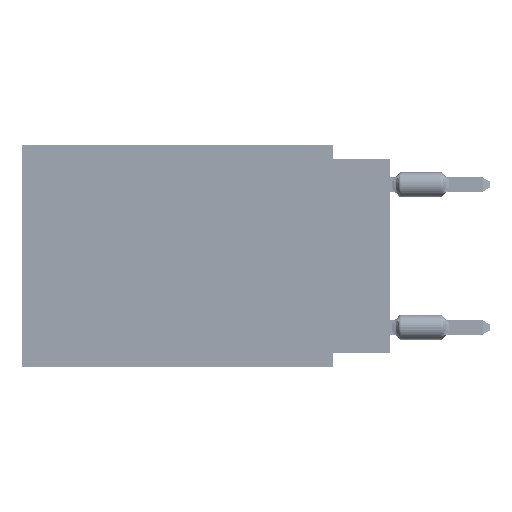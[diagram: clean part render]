
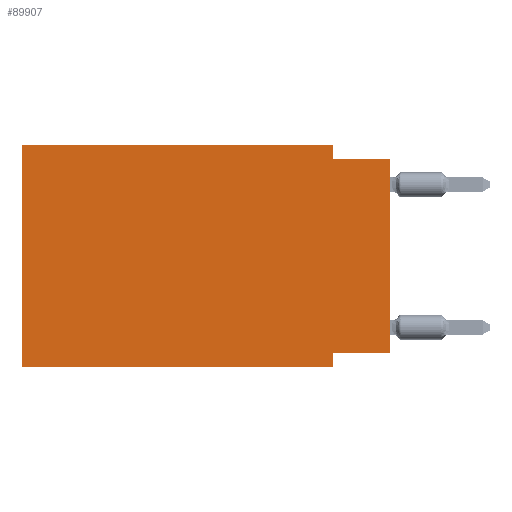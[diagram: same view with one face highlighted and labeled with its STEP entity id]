
A CAD part, left-side view. The second image highlights one B-rep face of the part: STEP entity #89907.
In plain terms, the highlighted planar face has unit normal (-1, 0, 0).
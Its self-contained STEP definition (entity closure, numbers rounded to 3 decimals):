
#1405 = LINE ( 'NONE', #71544, #45225 ) ;
#1411 = CARTESIAN_POINT ( 'NONE',  ( 0., 2.54, -9.906 ) ) ;
#1851 = AXIS2_PLACEMENT_3D ( 'NONE', #86816, #78167, #9817 ) ;
#9817 = DIRECTION ( 'NONE',  ( 0., 0., -1. ) ) ;
#9855 = ORIENTED_EDGE ( 'NONE', *, *, #84044, .T. ) ;
#11608 = ORIENTED_EDGE ( 'NONE', *, *, #20546, .T. ) ;
#14075 = VERTEX_POINT ( 'NONE', #1411 ) ;
#14467 = DIRECTION ( 'NONE',  ( 0., 0., 1. ) ) ;
#15139 = VECTOR ( 'NONE', #46938, 1000. ) ;
#15737 = VERTEX_POINT ( 'NONE', #35145 ) ;
#16542 = ORIENTED_EDGE ( 'NONE', *, *, #52613, .F. ) ;
#17741 = LINE ( 'NONE', #72874, #49326 ) ;
#18715 = LINE ( 'NONE', #19161, #15139 ) ;
#19161 = CARTESIAN_POINT ( 'NONE',  ( 0., 2.54, 0. ) ) ;
#20546 = EDGE_CURVE ( 'NONE', #51513, #14075, #88664, .T. ) ;
#20823 = VERTEX_POINT ( 'NONE', #58097 ) ;
#21518 = DIRECTION ( 'NONE',  ( 0., 0., -1. ) ) ;
#21965 = LINE ( 'NONE', #42917, #78584 ) ;
#22818 = EDGE_CURVE ( 'NONE', #60749, #85610, #1405, .T. ) ;
#23262 = DIRECTION ( 'NONE',  ( 0., -1., 0. ) ) ;
#26639 = VERTEX_POINT ( 'NONE', #79595 ) ;
#27002 = CARTESIAN_POINT ( 'NONE',  ( 0., 16.383, 0. ) ) ;
#28291 = ORIENTED_EDGE ( 'NONE', *, *, #59258, .F. ) ;
#28511 = CARTESIAN_POINT ( 'NONE',  ( 0., 2.54, -0.635 ) ) ;
#30251 = EDGE_LOOP ( 'NONE', ( #9855, #84826, #80996, #77245, #28291, #11608, #16542, #58809 ) ) ;
#33290 = VECTOR ( 'NONE', #14467, 1000. ) ;
#33835 = LINE ( 'NONE', #27002, #82146 ) ;
#35109 = CARTESIAN_POINT ( 'NONE',  ( 0., 16.383, 0. ) ) ;
#35145 = CARTESIAN_POINT ( 'NONE',  ( 0., 0., -9.271 ) ) ;
#42917 = CARTESIAN_POINT ( 'NONE',  ( 0., 2.54, -9.906 ) ) ;
#45225 = VECTOR ( 'NONE', #23262, 1000. ) ;
#46938 = DIRECTION ( 'NONE',  ( 0., 0., -1. ) ) ;
#49326 = VECTOR ( 'NONE', #59668, 1000. ) ;
#50366 = FACE_OUTER_BOUND ( 'NONE', #30251, .T. ) ;
#50719 = DIRECTION ( 'NONE',  ( 0., -1., 0. ) ) ;
#51172 = CARTESIAN_POINT ( 'NONE',  ( 0., 16.383, 0. ) ) ;
#51513 = VERTEX_POINT ( 'NONE', #52484 ) ;
#51613 = LINE ( 'NONE', #51172, #52098 ) ;
#52098 = VECTOR ( 'NONE', #50719, 1000. ) ;
#52484 = CARTESIAN_POINT ( 'NONE',  ( 0., 16.383, -9.906 ) ) ;
#52613 = EDGE_CURVE ( 'NONE', #26639, #14075, #21965, .T. ) ;
#54063 = CARTESIAN_POINT ( 'NONE',  ( 0., 0., -0.635 ) ) ;
#54790 = DIRECTION ( 'NONE',  ( 0., 0., 1. ) ) ;
#57299 = LINE ( 'NONE', #63220, #33290 ) ;
#58097 = CARTESIAN_POINT ( 'NONE',  ( 0., 2.54, 0. ) ) ;
#58809 = ORIENTED_EDGE ( 'NONE', *, *, #66293, .F. ) ;
#59258 = EDGE_CURVE ( 'NONE', #51513, #60043, #33835, .T. ) ;
#59668 = DIRECTION ( 'NONE',  ( 0., 1., 0. ) ) ;
#59760 = VECTOR ( 'NONE', #74988, 1000. ) ;
#60043 = VERTEX_POINT ( 'NONE', #35109 ) ;
#60749 = VERTEX_POINT ( 'NONE', #28511 ) ;
#63220 = CARTESIAN_POINT ( 'NONE',  ( 0., 0., 0. ) ) ;
#66293 = EDGE_CURVE ( 'NONE', #15737, #26639, #17741, .T. ) ;
#71411 = EDGE_CURVE ( 'NONE', #60043, #20823, #51613, .T. ) ;
#71544 = CARTESIAN_POINT ( 'NONE',  ( 0., 0., -0.635 ) ) ;
#72874 = CARTESIAN_POINT ( 'NONE',  ( 0., 0., -9.271 ) ) ;
#74988 = DIRECTION ( 'NONE',  ( 0., -1., 0. ) ) ;
#77245 = ORIENTED_EDGE ( 'NONE', *, *, #71411, .F. ) ;
#78167 = DIRECTION ( 'NONE',  ( 1., 0., 0. ) ) ;
#78584 = VECTOR ( 'NONE', #21518, 1000. ) ;
#79073 = EDGE_CURVE ( 'NONE', #20823, #60749, #18715, .T. ) ;
#79595 = CARTESIAN_POINT ( 'NONE',  ( 0., 2.54, -9.271 ) ) ;
#80482 = CARTESIAN_POINT ( 'NONE',  ( 0., 16.383, -9.906 ) ) ;
#80996 = ORIENTED_EDGE ( 'NONE', *, *, #79073, .F. ) ;
#82146 = VECTOR ( 'NONE', #54790, 1000. ) ;
#84044 = EDGE_CURVE ( 'NONE', #15737, #85610, #57299, .T. ) ;
#84826 = ORIENTED_EDGE ( 'NONE', *, *, #22818, .F. ) ;
#85002 = PLANE ( 'NONE',  #1851 ) ;
#85610 = VERTEX_POINT ( 'NONE', #54063 ) ;
#86816 = CARTESIAN_POINT ( 'NONE',  ( 0., 16.383, 0. ) ) ;
#88664 = LINE ( 'NONE', #80482, #59760 ) ;
#89907 = ADVANCED_FACE ( 'NONE', ( #50366 ), #85002, .F. ) ;
